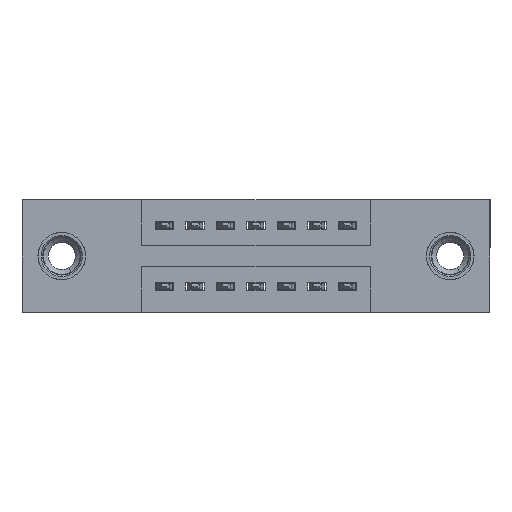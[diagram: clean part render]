
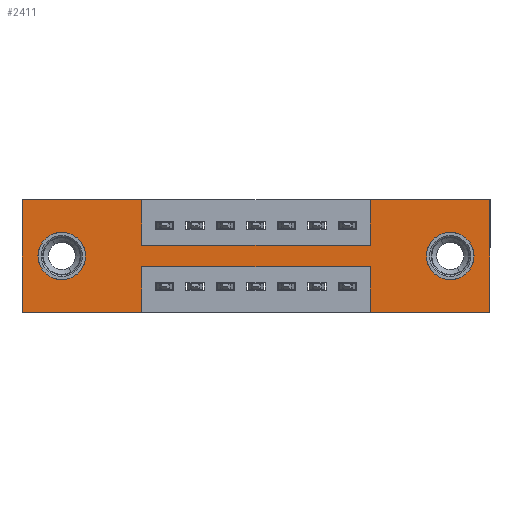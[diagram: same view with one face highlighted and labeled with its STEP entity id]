
A CAD part, front view. The second image highlights one B-rep face of the part: STEP entity #2411.
In plain terms, the highlighted planar face has unit normal (0, -1, 0).
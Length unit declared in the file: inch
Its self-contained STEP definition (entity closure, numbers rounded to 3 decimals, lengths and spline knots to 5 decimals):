
#261 = LINE ( 'NONE', #13467, #12297 ) ;
#816 = LINE ( 'NONE', #4672, #3930 ) ;
#971 = VERTEX_POINT ( 'NONE', #1542 ) ;
#1331 = LINE ( 'NONE', #9039, #10297 ) ;
#1367 = LINE ( 'NONE', #3487, #6897 ) ;
#1408 = ORIENTED_EDGE ( 'NONE', *, *, #12052, .F. ) ;
#1452 = VECTOR ( 'NONE', #3589, 39.37008 ) ;
#1478 = VERTEX_POINT ( 'NONE', #3500 ) ;
#1542 = CARTESIAN_POINT ( 'NONE',  ( 0.3925, 0., -0.22 ) ) ;
#1588 = AXIS2_PLACEMENT_3D ( 'NONE', #12040, #3908, #3859 ) ;
#1638 = VERTEX_POINT ( 'NONE', #2889 ) ;
#1662 = CARTESIAN_POINT ( 'NONE',  ( 1.1425, 0., 0. ) ) ;
#1884 = DIRECTION ( 'NONE',  ( -1., 0., 0. ) ) ;
#2340 = LINE ( 'NONE', #14649, #8209 ) ;
#2411 = ADVANCED_FACE ( 'NONE', ( #8169, #13549, #10513 ), #3922, .T. ) ;
#2588 = EDGE_CURVE ( 'NONE', #3179, #9201, #14805, .T. ) ;
#2889 = CARTESIAN_POINT ( 'NONE',  ( 1.535, 0., -0.37 ) ) ;
#2915 = VECTOR ( 'NONE', #14718, 39.37008 ) ;
#3043 = EDGE_CURVE ( 'NONE', #12680, #7483, #9415, .T. ) ;
#3119 = CARTESIAN_POINT ( 'NONE',  ( 1.405, 0., -0.185 ) ) ;
#3142 = VERTEX_POINT ( 'NONE', #9203 ) ;
#3155 = DIRECTION ( 'NONE',  ( 0., 0., 1. ) ) ;
#3179 = VERTEX_POINT ( 'NONE', #1662 ) ;
#3223 = DIRECTION ( 'NONE',  ( 0., 0., 1. ) ) ;
#3364 = EDGE_CURVE ( 'NONE', #13111, #8273, #14970, .T. ) ;
#3487 = CARTESIAN_POINT ( 'NONE',  ( 0., 0., -0.37 ) ) ;
#3500 = CARTESIAN_POINT ( 'NONE',  ( 1.405, 0., -0.107 ) ) ;
#3589 = DIRECTION ( 'NONE',  ( 1., 0., 0. ) ) ;
#3719 = EDGE_CURVE ( 'NONE', #4734, #3179, #1331, .T. ) ;
#3815 = VECTOR ( 'NONE', #7951, 39.37008 ) ;
#3859 = DIRECTION ( 'NONE',  ( 0., 0., -1. ) ) ;
#3908 = DIRECTION ( 'NONE',  ( 0., -1., 0. ) ) ;
#3922 = PLANE ( 'NONE',  #1588 ) ;
#3930 = VECTOR ( 'NONE', #11613, 39.37008 ) ;
#3957 = CARTESIAN_POINT ( 'NONE',  ( 1.405, 0., -0.263 ) ) ;
#4200 = CARTESIAN_POINT ( 'NONE',  ( 1.405, 0., -0.185 ) ) ;
#4265 = DIRECTION ( 'NONE',  ( 0., 0., -1. ) ) ;
#4307 = AXIS2_PLACEMENT_3D ( 'NONE', #6573, #14622, #7747 ) ;
#4319 = ORIENTED_EDGE ( 'NONE', *, *, #2588, .F. ) ;
#4369 = EDGE_LOOP ( 'NONE', ( #1408, #6668, #15077, #5091, #11214, #4319, #11182, #8116, #11989, #12978, #8880, #4602 ) ) ;
#4436 = EDGE_CURVE ( 'NONE', #7384, #4734, #8783, .T. ) ;
#4451 = ORIENTED_EDGE ( 'NONE', *, *, #3364, .T. ) ;
#4500 = VECTOR ( 'NONE', #12077, 39.37008 ) ;
#4602 = ORIENTED_EDGE ( 'NONE', *, *, #7720, .F. ) ;
#4643 = DIRECTION ( 'NONE',  ( -1., 0., 0. ) ) ;
#4672 = CARTESIAN_POINT ( 'NONE',  ( 0., 0., 0. ) ) ;
#4734 = VERTEX_POINT ( 'NONE', #14509 ) ;
#4833 = EDGE_CURVE ( 'NONE', #1638, #12680, #5668, .T. ) ;
#4860 = LINE ( 'NONE', #13308, #4500 ) ;
#4901 = CARTESIAN_POINT ( 'NONE',  ( 0.3925, 0., 0. ) ) ;
#5091 = ORIENTED_EDGE ( 'NONE', *, *, #4833, .F. ) ;
#5349 = VERTEX_POINT ( 'NONE', #3957 ) ;
#5384 = DIRECTION ( 'NONE',  ( 0., 0., -1. ) ) ;
#5550 = CARTESIAN_POINT ( 'NONE',  ( 0.13, 0., -0.185 ) ) ;
#5643 = DIRECTION ( 'NONE',  ( 1., 0., 0. ) ) ;
#5668 = LINE ( 'NONE', #6667, #2915 ) ;
#5961 = CARTESIAN_POINT ( 'NONE',  ( 0., 0., 0. ) ) ;
#6308 = VECTOR ( 'NONE', #11563, 39.37008 ) ;
#6357 = EDGE_CURVE ( 'NONE', #3142, #10791, #2340, .T. ) ;
#6385 = EDGE_CURVE ( 'NONE', #5349, #1478, #7845, .T. ) ;
#6573 = CARTESIAN_POINT ( 'NONE',  ( 0.13, 0., -0.185 ) ) ;
#6667 = CARTESIAN_POINT ( 'NONE',  ( 0., 0., -0.37 ) ) ;
#6668 = ORIENTED_EDGE ( 'NONE', *, *, #14286, .F. ) ;
#6897 = VECTOR ( 'NONE', #4643, 39.37008 ) ;
#7384 = VERTEX_POINT ( 'NONE', #12146 ) ;
#7483 = VERTEX_POINT ( 'NONE', #11156 ) ;
#7504 = EDGE_LOOP ( 'NONE', ( #12812, #12994 ) ) ;
#7505 = DIRECTION ( 'NONE',  ( 0., 1., 0. ) ) ;
#7720 = EDGE_CURVE ( 'NONE', #11160, #9780, #1367, .T. ) ;
#7747 = DIRECTION ( 'NONE',  ( 0., 0., 1. ) ) ;
#7773 = DIRECTION ( 'NONE',  ( 1., 0., 0. ) ) ;
#7845 = CIRCLE ( 'NONE', #14251, 0.078 ) ;
#7938 = CARTESIAN_POINT ( 'NONE',  ( 1.1425, 0., -0.37 ) ) ;
#7951 = DIRECTION ( 'NONE',  ( 0., 0., -1. ) ) ;
#7980 = CARTESIAN_POINT ( 'NONE',  ( 0.13, 0., -0.107 ) ) ;
#8116 = ORIENTED_EDGE ( 'NONE', *, *, #4436, .F. ) ;
#8169 = FACE_BOUND ( 'NONE', #7504, .T. ) ;
#8209 = VECTOR ( 'NONE', #7773, 39.37008 ) ;
#8273 = VERTEX_POINT ( 'NONE', #7980 ) ;
#8634 = CARTESIAN_POINT ( 'NONE',  ( 1.535, 0., 0. ) ) ;
#8695 = VECTOR ( 'NONE', #5643, 39.37008 ) ;
#8783 = LINE ( 'NONE', #10575, #1452 ) ;
#8880 = ORIENTED_EDGE ( 'NONE', *, *, #14934, .F. ) ;
#9039 = CARTESIAN_POINT ( 'NONE',  ( 1.1425, 0., 0. ) ) ;
#9201 = VERTEX_POINT ( 'NONE', #8634 ) ;
#9203 = CARTESIAN_POINT ( 'NONE',  ( 0., 0., 0. ) ) ;
#9415 = LINE ( 'NONE', #10745, #6308 ) ;
#9602 = CARTESIAN_POINT ( 'NONE',  ( 0.3925, 0., 0. ) ) ;
#9780 = VERTEX_POINT ( 'NONE', #9789 ) ;
#9789 = CARTESIAN_POINT ( 'NONE',  ( 0., 0., -0.37 ) ) ;
#10297 = VECTOR ( 'NONE', #3223, 39.37008 ) ;
#10513 = FACE_OUTER_BOUND ( 'NONE', #4369, .T. ) ;
#10575 = CARTESIAN_POINT ( 'NONE',  ( 0.3925, 0., -0.15 ) ) ;
#10745 = CARTESIAN_POINT ( 'NONE',  ( 1.1425, 0., -0.37 ) ) ;
#10749 = DIRECTION ( 'NONE',  ( 0., 0., -1. ) ) ;
#10791 = VERTEX_POINT ( 'NONE', #4901 ) ;
#11076 = CIRCLE ( 'NONE', #4307, 0.078 ) ;
#11156 = CARTESIAN_POINT ( 'NONE',  ( 1.1425, 0., -0.22 ) ) ;
#11160 = VERTEX_POINT ( 'NONE', #11337 ) ;
#11182 = ORIENTED_EDGE ( 'NONE', *, *, #3719, .F. ) ;
#11214 = ORIENTED_EDGE ( 'NONE', *, *, #14660, .F. ) ;
#11230 = DIRECTION ( 'NONE',  ( 0., 1., 0. ) ) ;
#11337 = CARTESIAN_POINT ( 'NONE',  ( 0.3925, 0., -0.37 ) ) ;
#11563 = DIRECTION ( 'NONE',  ( 0., 0., 1. ) ) ;
#11575 = EDGE_CURVE ( 'NONE', #1478, #5349, #12738, .T. ) ;
#11613 = DIRECTION ( 'NONE',  ( 0., 0., 1. ) ) ;
#11845 = ORIENTED_EDGE ( 'NONE', *, *, #13690, .T. ) ;
#11986 = VECTOR ( 'NONE', #10749, 39.37008 ) ;
#11989 = ORIENTED_EDGE ( 'NONE', *, *, #12900, .F. ) ;
#12040 = CARTESIAN_POINT ( 'NONE',  ( 0., 0., -0.37 ) ) ;
#12052 = EDGE_CURVE ( 'NONE', #971, #11160, #12724, .T. ) ;
#12077 = DIRECTION ( 'NONE',  ( 0., 0., -1. ) ) ;
#12146 = CARTESIAN_POINT ( 'NONE',  ( 0.3925, 0., -0.15 ) ) ;
#12297 = VECTOR ( 'NONE', #1884, 39.37008 ) ;
#12311 = DIRECTION ( 'NONE',  ( 0., 1., 0. ) ) ;
#12680 = VERTEX_POINT ( 'NONE', #7938 ) ;
#12724 = LINE ( 'NONE', #14833, #3815 ) ;
#12738 = CIRCLE ( 'NONE', #14777, 0.078 ) ;
#12812 = ORIENTED_EDGE ( 'NONE', *, *, #11575, .T. ) ;
#12900 = EDGE_CURVE ( 'NONE', #10791, #7384, #15058, .T. ) ;
#12978 = ORIENTED_EDGE ( 'NONE', *, *, #6357, .F. ) ;
#12994 = ORIENTED_EDGE ( 'NONE', *, *, #6385, .T. ) ;
#13111 = VERTEX_POINT ( 'NONE', #13305 ) ;
#13305 = CARTESIAN_POINT ( 'NONE',  ( 0.13, 0., -0.263 ) ) ;
#13308 = CARTESIAN_POINT ( 'NONE',  ( 1.535, 0., 0. ) ) ;
#13467 = CARTESIAN_POINT ( 'NONE',  ( 0.3925, 0., -0.22 ) ) ;
#13549 = FACE_BOUND ( 'NONE', #14034, .T. ) ;
#13690 = EDGE_CURVE ( 'NONE', #8273, #13111, #11076, .T. ) ;
#14034 = EDGE_LOOP ( 'NONE', ( #11845, #4451 ) ) ;
#14251 = AXIS2_PLACEMENT_3D ( 'NONE', #3119, #11230, #4265 ) ;
#14286 = EDGE_CURVE ( 'NONE', #7483, #971, #261, .T. ) ;
#14509 = CARTESIAN_POINT ( 'NONE',  ( 1.1425, 0., -0.15 ) ) ;
#14511 = AXIS2_PLACEMENT_3D ( 'NONE', #5550, #7505, #3155 ) ;
#14622 = DIRECTION ( 'NONE',  ( 0., 1., 0. ) ) ;
#14649 = CARTESIAN_POINT ( 'NONE',  ( 0., 0., 0. ) ) ;
#14660 = EDGE_CURVE ( 'NONE', #9201, #1638, #4860, .T. ) ;
#14718 = DIRECTION ( 'NONE',  ( -1., 0., 0. ) ) ;
#14777 = AXIS2_PLACEMENT_3D ( 'NONE', #4200, #12311, #5384 ) ;
#14805 = LINE ( 'NONE', #5961, #8695 ) ;
#14833 = CARTESIAN_POINT ( 'NONE',  ( 0.3925, 0., -0.37 ) ) ;
#14934 = EDGE_CURVE ( 'NONE', #9780, #3142, #816, .T. ) ;
#14970 = CIRCLE ( 'NONE', #14511, 0.078 ) ;
#15058 = LINE ( 'NONE', #9602, #11986 ) ;
#15077 = ORIENTED_EDGE ( 'NONE', *, *, #3043, .F. ) ;
